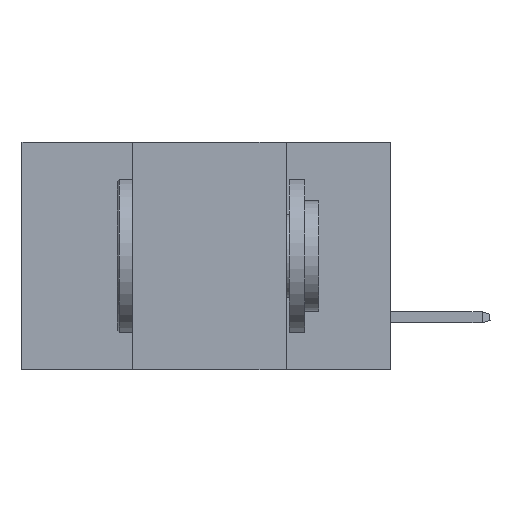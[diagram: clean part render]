
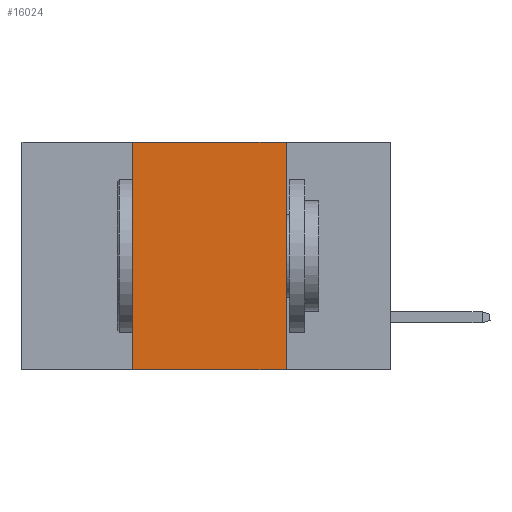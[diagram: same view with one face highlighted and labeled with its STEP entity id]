
A CAD part, left-side view. The second image highlights one B-rep face of the part: STEP entity #16024.
In plain terms, the highlighted planar face has unit normal (-1, 0, 0).
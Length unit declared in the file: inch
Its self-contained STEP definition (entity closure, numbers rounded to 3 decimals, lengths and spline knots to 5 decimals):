
#1116 = VECTOR ( 'NONE', #2079, 39.37008 ) ;
#1378 = EDGE_CURVE ( 'NONE', #2243, #17001, #12191, .T. ) ;
#2079 = DIRECTION ( 'NONE',  ( 0., 0., 1. ) ) ;
#2243 = VERTEX_POINT ( 'NONE', #9422 ) ;
#2352 = AXIS2_PLACEMENT_3D ( 'NONE', #6273, #9711, #4675 ) ;
#3098 = DIRECTION ( 'NONE',  ( 0., -1., 0. ) ) ;
#4346 = EDGE_CURVE ( 'NONE', #2243, #4862, #20170, .T. ) ;
#4625 = ORIENTED_EDGE ( 'NONE', *, *, #4346, .F. ) ;
#4675 = DIRECTION ( 'NONE',  ( 0., 0., -1. ) ) ;
#4862 = VERTEX_POINT ( 'NONE', #5391 ) ;
#5283 = VERTEX_POINT ( 'NONE', #13873 ) ;
#5391 = CARTESIAN_POINT ( 'NONE',  ( 0., 0.42, 0. ) ) ;
#5439 = CARTESIAN_POINT ( 'NONE',  ( 0., 0.6, -0.37 ) ) ;
#6273 = CARTESIAN_POINT ( 'NONE',  ( 0., 0.6, 0. ) ) ;
#6995 = VECTOR ( 'NONE', #17305, 39.37008 ) ;
#7596 = FACE_OUTER_BOUND ( 'NONE', #17209, .T. ) ;
#8265 = CARTESIAN_POINT ( 'NONE',  ( 0., 0.6, 0. ) ) ;
#8755 = CARTESIAN_POINT ( 'NONE',  ( 0., 0.17, -0.37 ) ) ;
#8913 = EDGE_CURVE ( 'NONE', #4862, #5283, #20300, .T. ) ;
#9422 = CARTESIAN_POINT ( 'NONE',  ( 0., 0.42, -0.37 ) ) ;
#9711 = DIRECTION ( 'NONE',  ( 1., 0., 0. ) ) ;
#12191 = LINE ( 'NONE', #5439, #20321 ) ;
#12528 = CARTESIAN_POINT ( 'NONE',  ( 0., 0.42, 0. ) ) ;
#12892 = ORIENTED_EDGE ( 'NONE', *, *, #1378, .T. ) ;
#13814 = CARTESIAN_POINT ( 'NONE',  ( 0., 0.17, 0. ) ) ;
#13823 = VECTOR ( 'NONE', #3098, 39.37008 ) ;
#13873 = CARTESIAN_POINT ( 'NONE',  ( 0., 0.17, 0. ) ) ;
#15124 = PLANE ( 'NONE',  #2352 ) ;
#15625 = ORIENTED_EDGE ( 'NONE', *, *, #16963, .F. ) ;
#16006 = LINE ( 'NONE', #13814, #6995 ) ;
#16024 = ADVANCED_FACE ( 'NONE', ( #7596 ), #15124, .F. ) ;
#16963 = EDGE_CURVE ( 'NONE', #5283, #17001, #16006, .T. ) ;
#17001 = VERTEX_POINT ( 'NONE', #8755 ) ;
#17209 = EDGE_LOOP ( 'NONE', ( #15625, #20522, #4625, #12892 ) ) ;
#17305 = DIRECTION ( 'NONE',  ( 0., 0., -1. ) ) ;
#20170 = LINE ( 'NONE', #12528, #1116 ) ;
#20300 = LINE ( 'NONE', #8265, #13823 ) ;
#20321 = VECTOR ( 'NONE', #21012, 39.37008 ) ;
#20522 = ORIENTED_EDGE ( 'NONE', *, *, #8913, .F. ) ;
#21012 = DIRECTION ( 'NONE',  ( 0., -1., 0. ) ) ;
